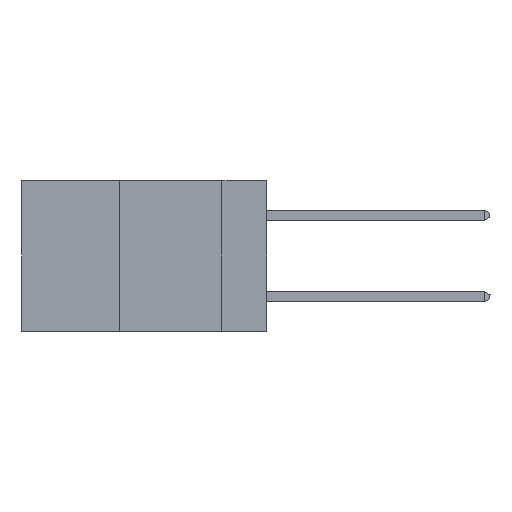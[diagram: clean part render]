
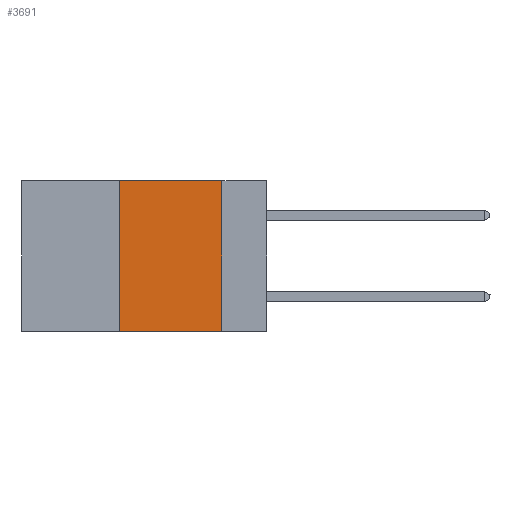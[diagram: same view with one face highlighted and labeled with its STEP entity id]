
A CAD part, left-side view. The second image highlights one B-rep face of the part: STEP entity #3691.
In plain terms, the highlighted planar face has unit normal (-1, 0, 0).
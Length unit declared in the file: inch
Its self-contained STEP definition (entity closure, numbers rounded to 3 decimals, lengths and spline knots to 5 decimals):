
#104 = CARTESIAN_POINT ( 'NONE',  ( 0., 0.36, -0.37 ) ) ;
#261 = LINE ( 'NONE', #27982, #36947 ) ;
#603 = ORIENTED_EDGE ( 'NONE', *, *, #14398, .F. ) ;
#1467 = VECTOR ( 'NONE', #17183, 39.37008 ) ;
#1913 = DIRECTION ( 'NONE',  ( 0., -1., 0. ) ) ;
#2966 = EDGE_CURVE ( 'NONE', #18913, #37084, #261, .T. ) ;
#3691 = ADVANCED_FACE ( 'NONE', ( #21786 ), #28872, .F. ) ;
#4820 = EDGE_CURVE ( 'NONE', #36327, #18913, #7051, .T. ) ;
#7051 = LINE ( 'NONE', #44254, #16275 ) ;
#8480 = DIRECTION ( 'NONE',  ( 1., 0., 0. ) ) ;
#9028 = CARTESIAN_POINT ( 'NONE',  ( 0., 0.11, -0.37 ) ) ;
#12202 = CARTESIAN_POINT ( 'NONE',  ( 0., 0.6, -0.37 ) ) ;
#12911 = ORIENTED_EDGE ( 'NONE', *, *, #43469, .T. ) ;
#13703 = LINE ( 'NONE', #12202, #20762 ) ;
#14398 = EDGE_CURVE ( 'NONE', #37084, #16884, #20383, .T. ) ;
#14635 = ORIENTED_EDGE ( 'NONE', *, *, #4820, .F. ) ;
#16275 = VECTOR ( 'NONE', #41223, 39.37008 ) ;
#16884 = VERTEX_POINT ( 'NONE', #9028 ) ;
#17183 = DIRECTION ( 'NONE',  ( 0., 0., -1. ) ) ;
#18913 = VERTEX_POINT ( 'NONE', #41635 ) ;
#20383 = LINE ( 'NONE', #31193, #1467 ) ;
#20702 = ORIENTED_EDGE ( 'NONE', *, *, #2966, .F. ) ;
#20762 = VECTOR ( 'NONE', #1913, 39.37008 ) ;
#21657 = DIRECTION ( 'NONE',  ( 0., 0., -1. ) ) ;
#21786 = FACE_OUTER_BOUND ( 'NONE', #33011, .T. ) ;
#27562 = AXIS2_PLACEMENT_3D ( 'NONE', #35823, #8480, #21657 ) ;
#27982 = CARTESIAN_POINT ( 'NONE',  ( 0., 0.6, 0. ) ) ;
#28872 = PLANE ( 'NONE',  #27562 ) ;
#31193 = CARTESIAN_POINT ( 'NONE',  ( 0., 0.11, 0. ) ) ;
#33011 = EDGE_LOOP ( 'NONE', ( #603, #20702, #14635, #12911 ) ) ;
#35823 = CARTESIAN_POINT ( 'NONE',  ( 0., 0.6, 0. ) ) ;
#36327 = VERTEX_POINT ( 'NONE', #104 ) ;
#36947 = VECTOR ( 'NONE', #37948, 39.37008 ) ;
#37084 = VERTEX_POINT ( 'NONE', #38555 ) ;
#37948 = DIRECTION ( 'NONE',  ( 0., -1., 0. ) ) ;
#38555 = CARTESIAN_POINT ( 'NONE',  ( 0., 0.11, 0. ) ) ;
#41223 = DIRECTION ( 'NONE',  ( 0., 0., 1. ) ) ;
#41635 = CARTESIAN_POINT ( 'NONE',  ( 0., 0.36, 0. ) ) ;
#43469 = EDGE_CURVE ( 'NONE', #36327, #16884, #13703, .T. ) ;
#44254 = CARTESIAN_POINT ( 'NONE',  ( 0., 0.36, 0. ) ) ;
